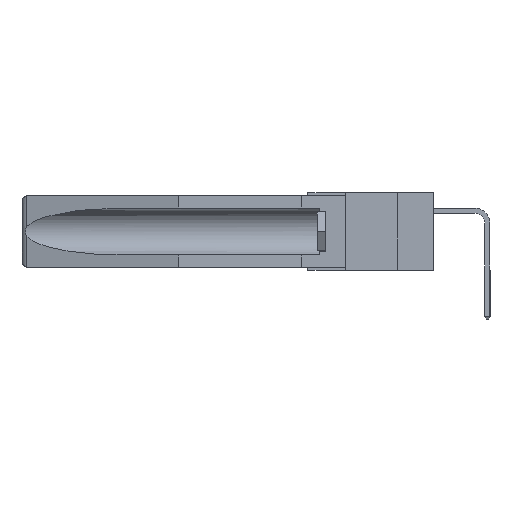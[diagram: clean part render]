
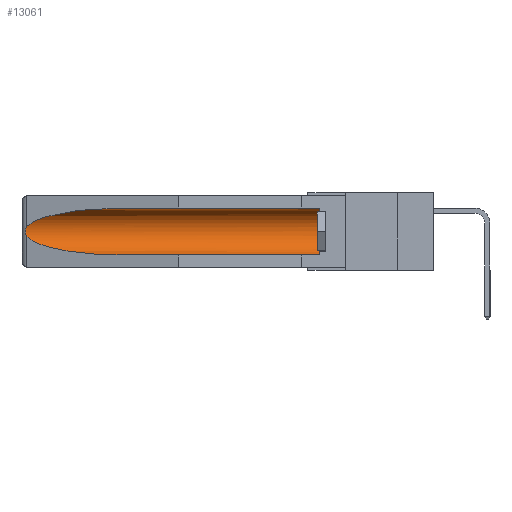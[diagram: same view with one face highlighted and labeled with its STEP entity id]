
A CAD part, left-side view. The second image highlights one B-rep face of the part: STEP entity #13061.
In plain terms, the highlighted cylindrical face has radius 2.857 mm (diameter 5.715 mm), a partial arc.
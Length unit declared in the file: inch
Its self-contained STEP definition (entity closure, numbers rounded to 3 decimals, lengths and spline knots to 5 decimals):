
#850 = CARTESIAN_POINT ( 'NONE',  ( 0.26655, 1.53094, -0.18657 ) ) ;
#935 = CARTESIAN_POINT ( 'NONE',  ( 0.155, -0.30754, -0.284 ) ) ;
#1119 = CARTESIAN_POINT ( 'NONE',  ( 0.2673, 1.5327, -0.16383 ) ) ;
#2054 = CARTESIAN_POINT ( 'NONE',  ( 0.26537, 1.52718, -0.14972 ) ) ;
#2228 = CARTESIAN_POINT ( 'NONE',  ( 0.21114, 1.30732, -0.059 ) ) ;
#3074 = AXIS2_PLACEMENT_3D ( 'NONE', #18510, #12104, #27138 ) ;
#3245 = CARTESIAN_POINT ( 'NONE',  ( 0.2673, 1.53269, -0.17917 ) ) ;
#3519 = ORIENTED_EDGE ( 'NONE', *, *, #26613, .T. ) ;
#4570 = AXIS2_PLACEMENT_3D ( 'NONE', #23371, #25630, #7133 ) ;
#4698 = VERTEX_POINT ( 'NONE', #27349 ) ;
#5000 = CARTESIAN_POINT ( 'NONE',  ( 0.155, 1.07973, -0.284 ) ) ;
#5133 = CARTESIAN_POINT ( 'NONE',  ( 0.26654, 1.53092, -0.15636 ) ) ;
#5241 = ORIENTED_EDGE ( 'NONE', *, *, #10013, .T. ) ;
#5971 = EDGE_LOOP ( 'NONE', ( #15551, #19019, #15159, #19440, #5241, #3519 ) ) ;
#6648 =( BOUNDED_CURVE ( )  B_SPLINE_CURVE ( 3, ( #25839, #2228, #17218, #2054 ),
 .UNSPECIFIED., .F., .F. ) 
 B_SPLINE_CURVE_WITH_KNOTS ( ( 4, 4 ),
 ( 4.71239, 6.08839 ),
 .UNSPECIFIED. ) 
 CURVE ( )  GEOMETRIC_REPRESENTATION_ITEM ( )  RATIONAL_B_SPLINE_CURVE ( ( 1., 0.848, 0.848, 1. ) ) 
 REPRESENTATION_ITEM ( '' )  );
#7133 = DIRECTION ( 'NONE',  ( 0., 0., 1. ) ) ;
#7191 = CARTESIAN_POINT ( 'NONE',  ( 0.155, 0.126, -0.059 ) ) ;
#8654 = VERTEX_POINT ( 'NONE', #7191 ) ;
#8953 = CARTESIAN_POINT ( 'NONE',  ( 0.26537, 1.52718, -0.19328 ) ) ;
#9376 = CARTESIAN_POINT ( 'NONE',  ( 0.155, 0.126, -0.284 ) ) ;
#10013 = EDGE_CURVE ( 'NONE', #10096, #8654, #23284, .T. ) ;
#10096 = VERTEX_POINT ( 'NONE', #9376 ) ;
#10469 = VECTOR ( 'NONE', #16102, 39.37008 ) ;
#10790 = EDGE_CURVE ( 'NONE', #10096, #12804, #11136, .T. ) ;
#11136 = LINE ( 'NONE', #935, #10469 ) ;
#12104 = DIRECTION ( 'NONE',  ( 0., -1., 0. ) ) ;
#12804 = VERTEX_POINT ( 'NONE', #21050 ) ;
#13061 = ADVANCED_FACE ( 'NONE', ( #24789 ), #22111, .F. ) ;
#13550 = CARTESIAN_POINT ( 'NONE',  ( 0.26537, 1.52718, -0.14972 ) ) ;
#13668 =( BOUNDED_CURVE ( )  B_SPLINE_CURVE ( 3, ( #8953, #15417, #20018, #5000 ),
 .UNSPECIFIED., .F., .F. ) 
 B_SPLINE_CURVE_WITH_KNOTS ( ( 4, 4 ),
 ( 0.1948, 1.5708 ),
 .UNSPECIFIED. ) 
 CURVE ( )  GEOMETRIC_REPRESENTATION_ITEM ( )  RATIONAL_B_SPLINE_CURVE ( ( 1., 0.848, 0.848, 1. ) ) 
 REPRESENTATION_ITEM ( '' )  );
#13779 = CARTESIAN_POINT ( 'NONE',  ( 0.155, -0.30754, -0.059 ) ) ;
#14384 = VERTEX_POINT ( 'NONE', #20784 ) ;
#15159 = ORIENTED_EDGE ( 'NONE', *, *, #24796, .T. ) ;
#15417 = CARTESIAN_POINT ( 'NONE',  ( 0.25451, 1.48313, -0.24835 ) ) ;
#15551 = ORIENTED_EDGE ( 'NONE', *, *, #26745, .T. ) ;
#15832 = CARTESIAN_POINT ( 'NONE',  ( 0.26597, 1.5296, -0.19026 ) ) ;
#15929 = CARTESIAN_POINT ( 'NONE',  ( 0.26537, 1.52718, -0.14972 ) ) ;
#16102 = DIRECTION ( 'NONE',  ( 0., 1., 0. ) ) ;
#17218 = CARTESIAN_POINT ( 'NONE',  ( 0.25451, 1.48313, -0.09465 ) ) ;
#17534 = EDGE_CURVE ( 'NONE', #25899, #4698, #26233, .T. ) ;
#18307 = VECTOR ( 'NONE', #26922, 39.37008 ) ;
#18510 = CARTESIAN_POINT ( 'NONE',  ( 0.155, 0.126, -0.1715 ) ) ;
#19019 = ORIENTED_EDGE ( 'NONE', *, *, #17534, .T. ) ;
#19440 = ORIENTED_EDGE ( 'NONE', *, *, #10790, .F. ) ;
#20018 = CARTESIAN_POINT ( 'NONE',  ( 0.21114, 1.30732, -0.284 ) ) ;
#20324 = LINE ( 'NONE', #13779, #18307 ) ;
#20419 = CARTESIAN_POINT ( 'NONE',  ( 0.26597, 1.52961, -0.15275 ) ) ;
#20784 = CARTESIAN_POINT ( 'NONE',  ( 0.155, 1.07973, -0.059 ) ) ;
#21050 = CARTESIAN_POINT ( 'NONE',  ( 0.155, 1.07973, -0.284 ) ) ;
#22111 = CYLINDRICAL_SURFACE ( 'NONE', #4570, 0.1125 ) ;
#22565 = CARTESIAN_POINT ( 'NONE',  ( 0.2675, 1.53308, -0.16763 ) ) ;
#22650 = CARTESIAN_POINT ( 'NONE',  ( 0.26537, 1.52718, -0.19328 ) ) ;
#23284 = CIRCLE ( 'NONE', #3074, 0.1125 ) ;
#23371 = CARTESIAN_POINT ( 'NONE',  ( 0.155, -0.30754, -0.1715 ) ) ;
#24622 = CARTESIAN_POINT ( 'NONE',  ( 0.2675, 1.53308, -0.17534 ) ) ;
#24789 = FACE_OUTER_BOUND ( 'NONE', #5971, .T. ) ;
#24796 = EDGE_CURVE ( 'NONE', #4698, #12804, #13668, .T. ) ;
#25630 = DIRECTION ( 'NONE',  ( 0., 1., 0. ) ) ;
#25839 = CARTESIAN_POINT ( 'NONE',  ( 0.155, 1.07973, -0.059 ) ) ;
#25899 = VERTEX_POINT ( 'NONE', #13550 ) ;
#26233 = B_SPLINE_CURVE_WITH_KNOTS ( 'NONE', 3,
 ( #15929, #20419, #5133, #1119, #22565, #24622, #3245, #850, #15832, #22650 ),
 .UNSPECIFIED., .F., .F.,
 ( 4, 2, 2, 2, 4 ),
 ( 0., 0.00029, 0.00058, 0.00087, 0.00117 ),
 .UNSPECIFIED. ) ;
#26613 = EDGE_CURVE ( 'NONE', #8654, #14384, #20324, .T. ) ;
#26745 = EDGE_CURVE ( 'NONE', #14384, #25899, #6648, .T. ) ;
#26922 = DIRECTION ( 'NONE',  ( 0., 1., 0. ) ) ;
#27138 = DIRECTION ( 'NONE',  ( 0., 0., 1. ) ) ;
#27349 = CARTESIAN_POINT ( 'NONE',  ( 0.26537, 1.52718, -0.19328 ) ) ;
